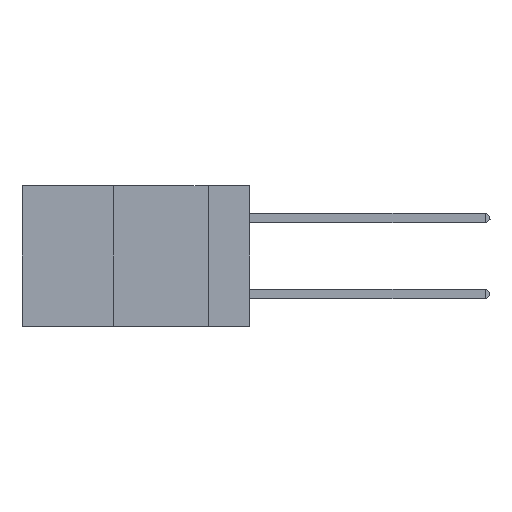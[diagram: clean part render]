
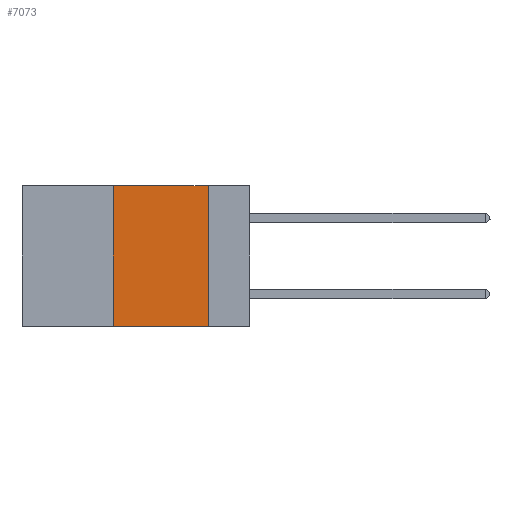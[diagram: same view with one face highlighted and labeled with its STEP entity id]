
A CAD part, left-side view. The second image highlights one B-rep face of the part: STEP entity #7073.
In plain terms, the highlighted planar face has unit normal (-1, 0, 0).
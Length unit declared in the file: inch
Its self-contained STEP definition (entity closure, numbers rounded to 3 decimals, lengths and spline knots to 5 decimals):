
#44 = PLANE ( 'NONE',  #2207 ) ;
#331 = LINE ( 'NONE', #10224, #1125 ) ;
#594 = ORIENTED_EDGE ( 'NONE', *, *, #13440, .F. ) ;
#1050 = VECTOR ( 'NONE', #15312, 39.37008 ) ;
#1125 = VECTOR ( 'NONE', #12489, 39.37008 ) ;
#1181 = VERTEX_POINT ( 'NONE', #14045 ) ;
#1186 = FACE_OUTER_BOUND ( 'NONE', #13973, .T. ) ;
#1654 = CARTESIAN_POINT ( 'NONE',  ( 0., 0.36, 0. ) ) ;
#2207 = AXIS2_PLACEMENT_3D ( 'NONE', #3793, #12444, #8717 ) ;
#2872 = ORIENTED_EDGE ( 'NONE', *, *, #3468, .F. ) ;
#2979 = CARTESIAN_POINT ( 'NONE',  ( 0., 0.6, -0.37 ) ) ;
#3468 = EDGE_CURVE ( 'NONE', #10908, #9262, #8337, .T. ) ;
#3793 = CARTESIAN_POINT ( 'NONE',  ( 0., 0.6, 0. ) ) ;
#5384 = CARTESIAN_POINT ( 'NONE',  ( 0., 0.36, 0. ) ) ;
#5466 = EDGE_CURVE ( 'NONE', #1181, #8262, #14054, .T. ) ;
#5914 = DIRECTION ( 'NONE',  ( 0., -1., 0. ) ) ;
#7073 = ADVANCED_FACE ( 'NONE', ( #1186 ), #44, .F. ) ;
#7903 = DIRECTION ( 'NONE',  ( 0., -1., 0. ) ) ;
#8262 = VERTEX_POINT ( 'NONE', #14241 ) ;
#8263 = CARTESIAN_POINT ( 'NONE',  ( 0., 0.6, 0. ) ) ;
#8337 = LINE ( 'NONE', #8263, #13956 ) ;
#8717 = DIRECTION ( 'NONE',  ( 0., 0., -1. ) ) ;
#9262 = VERTEX_POINT ( 'NONE', #9831 ) ;
#9382 = EDGE_CURVE ( 'NONE', #9262, #8262, #331, .T. ) ;
#9831 = CARTESIAN_POINT ( 'NONE',  ( 0., 0.11, 0. ) ) ;
#10224 = CARTESIAN_POINT ( 'NONE',  ( 0., 0.11, 0. ) ) ;
#10838 = ORIENTED_EDGE ( 'NONE', *, *, #9382, .F. ) ;
#10908 = VERTEX_POINT ( 'NONE', #5384 ) ;
#12444 = DIRECTION ( 'NONE',  ( 1., 0., 0. ) ) ;
#12489 = DIRECTION ( 'NONE',  ( 0., 0., -1. ) ) ;
#13440 = EDGE_CURVE ( 'NONE', #1181, #10908, #14100, .T. ) ;
#13956 = VECTOR ( 'NONE', #5914, 39.37008 ) ;
#13965 = ORIENTED_EDGE ( 'NONE', *, *, #5466, .T. ) ;
#13973 = EDGE_LOOP ( 'NONE', ( #10838, #2872, #594, #13965 ) ) ;
#14045 = CARTESIAN_POINT ( 'NONE',  ( 0., 0.36, -0.37 ) ) ;
#14054 = LINE ( 'NONE', #2979, #14560 ) ;
#14100 = LINE ( 'NONE', #1654, #1050 ) ;
#14241 = CARTESIAN_POINT ( 'NONE',  ( 0., 0.11, -0.37 ) ) ;
#14560 = VECTOR ( 'NONE', #7903, 39.37008 ) ;
#15312 = DIRECTION ( 'NONE',  ( 0., 0., 1. ) ) ;
